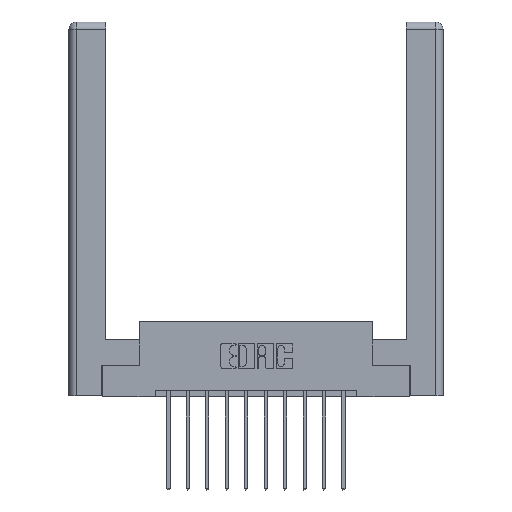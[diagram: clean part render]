
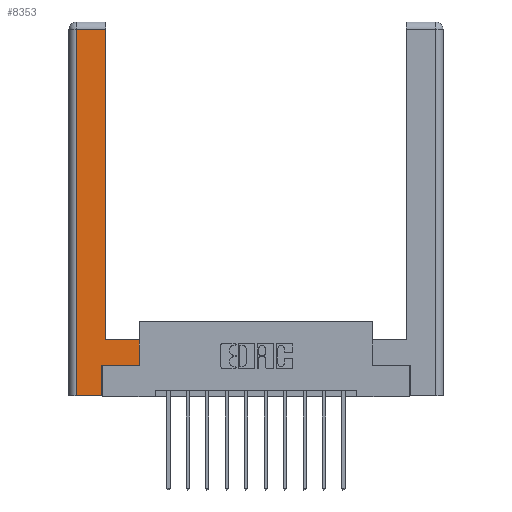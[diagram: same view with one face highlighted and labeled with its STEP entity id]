
A CAD part, top view. The second image highlights one B-rep face of the part: STEP entity #8353.
In plain terms, the highlighted planar face has unit normal (0, 0, 1).
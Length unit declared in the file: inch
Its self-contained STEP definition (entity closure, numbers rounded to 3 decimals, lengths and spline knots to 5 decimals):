
#63 = EDGE_LOOP ( 'NONE', ( #5025, #578, #2762, #4601, #14393, #1613, #6290, #5236 ) ) ;
#109 = DIRECTION ( 'NONE',  ( 0., 1., 0. ) ) ;
#138 = DIRECTION ( 'NONE',  ( 0., 1., 0. ) ) ;
#261 = DIRECTION ( 'NONE',  ( 1., 0., 0. ) ) ;
#522 = LINE ( 'NONE', #3432, #3669 ) ;
#578 = ORIENTED_EDGE ( 'NONE', *, *, #1402, .T. ) ;
#630 = VECTOR ( 'NONE', #9460, 39.37008 ) ;
#1001 = VECTOR ( 'NONE', #12050, 39.37008 ) ;
#1402 = EDGE_CURVE ( 'NONE', #11550, #8214, #7752, .T. ) ;
#1460 = CARTESIAN_POINT ( 'NONE',  ( 0.295, 0.45, 0. ) ) ;
#1613 = ORIENTED_EDGE ( 'NONE', *, *, #5504, .T. ) ;
#1838 = VECTOR ( 'NONE', #261, 39.37008 ) ;
#2034 = EDGE_CURVE ( 'NONE', #13854, #13527, #8766, .T. ) ;
#2553 = DIRECTION ( 'NONE',  ( -1., 0., 0. ) ) ;
#2762 = ORIENTED_EDGE ( 'NONE', *, *, #7700, .T. ) ;
#3165 = CARTESIAN_POINT ( 'NONE',  ( 0.265, 0., 0. ) ) ;
#3342 = CARTESIAN_POINT ( 'NONE',  ( 0.295, 3., 0. ) ) ;
#3417 = LINE ( 'NONE', #1460, #630 ) ;
#3432 = CARTESIAN_POINT ( 'NONE',  ( 0.565, 0.45, 0. ) ) ;
#3496 = CARTESIAN_POINT ( 'NONE',  ( 0.565, 0.245, 0. ) ) ;
#3533 = CARTESIAN_POINT ( 'NONE',  ( 0.0615, 2.94, 0. ) ) ;
#3669 = VECTOR ( 'NONE', #9099, 39.37008 ) ;
#3971 = CARTESIAN_POINT ( 'NONE',  ( 0.265, 0., 0. ) ) ;
#4296 = EDGE_CURVE ( 'NONE', #12742, #10742, #3417, .T. ) ;
#4601 = ORIENTED_EDGE ( 'NONE', *, *, #2034, .T. ) ;
#4670 = LINE ( 'NONE', #13049, #1001 ) ;
#4838 = CARTESIAN_POINT ( 'NONE',  ( 0.0615, 2.94, 0. ) ) ;
#5025 = ORIENTED_EDGE ( 'NONE', *, *, #7947, .T. ) ;
#5092 = VECTOR ( 'NONE', #138, 39.37008 ) ;
#5236 = ORIENTED_EDGE ( 'NONE', *, *, #4296, .T. ) ;
#5504 = EDGE_CURVE ( 'NONE', #6971, #14296, #6433, .T. ) ;
#5988 = PLANE ( 'NONE',  #8717 ) ;
#6191 = CARTESIAN_POINT ( 'NONE',  ( 0.295, 0.45, 0. ) ) ;
#6290 = ORIENTED_EDGE ( 'NONE', *, *, #12501, .T. ) ;
#6350 = CARTESIAN_POINT ( 'NONE',  ( 0.0615, 0., 0. ) ) ;
#6433 = LINE ( 'NONE', #13715, #1838 ) ;
#6971 = VERTEX_POINT ( 'NONE', #14559 ) ;
#6976 = FACE_OUTER_BOUND ( 'NONE', #63, .T. ) ;
#7532 = LINE ( 'NONE', #3342, #7866 ) ;
#7700 = EDGE_CURVE ( 'NONE', #8214, #13854, #4670, .T. ) ;
#7752 = LINE ( 'NONE', #4838, #8796 ) ;
#7866 = VECTOR ( 'NONE', #109, 39.37008 ) ;
#7947 = EDGE_CURVE ( 'NONE', #10742, #11550, #7532, .T. ) ;
#8214 = VERTEX_POINT ( 'NONE', #3533 ) ;
#8335 = CARTESIAN_POINT ( 'NONE',  ( 0.295, 2.94, 0. ) ) ;
#8353 = ADVANCED_FACE ( 'NONE', ( #6976 ), #5988, .F. ) ;
#8717 = AXIS2_PLACEMENT_3D ( 'NONE', #10618, #11653, #2553 ) ;
#8766 = LINE ( 'NONE', #3971, #13172 ) ;
#8796 = VECTOR ( 'NONE', #14194, 39.37008 ) ;
#9099 = DIRECTION ( 'NONE',  ( 0., 1., 0. ) ) ;
#9460 = DIRECTION ( 'NONE',  ( -1., 0., 0. ) ) ;
#10618 = CARTESIAN_POINT ( 'NONE',  ( 0., 0., 0. ) ) ;
#10742 = VERTEX_POINT ( 'NONE', #6191 ) ;
#11064 = LINE ( 'NONE', #12473, #5092 ) ;
#11550 = VERTEX_POINT ( 'NONE', #8335 ) ;
#11653 = DIRECTION ( 'NONE',  ( 0., 0., -1. ) ) ;
#12050 = DIRECTION ( 'NONE',  ( 0., -1., 0. ) ) ;
#12283 = EDGE_CURVE ( 'NONE', #13527, #6971, #11064, .T. ) ;
#12473 = CARTESIAN_POINT ( 'NONE',  ( 0.265, 0.245, 0. ) ) ;
#12501 = EDGE_CURVE ( 'NONE', #14296, #12742, #522, .T. ) ;
#12742 = VERTEX_POINT ( 'NONE', #14515 ) ;
#13049 = CARTESIAN_POINT ( 'NONE',  ( 0.0615, 0., 0. ) ) ;
#13172 = VECTOR ( 'NONE', #13177, 39.37008 ) ;
#13177 = DIRECTION ( 'NONE',  ( 1., 0., 0. ) ) ;
#13527 = VERTEX_POINT ( 'NONE', #3165 ) ;
#13715 = CARTESIAN_POINT ( 'NONE',  ( 0.565, 0.245, 0. ) ) ;
#13854 = VERTEX_POINT ( 'NONE', #6350 ) ;
#14194 = DIRECTION ( 'NONE',  ( -1., 0., 0. ) ) ;
#14296 = VERTEX_POINT ( 'NONE', #3496 ) ;
#14393 = ORIENTED_EDGE ( 'NONE', *, *, #12283, .T. ) ;
#14515 = CARTESIAN_POINT ( 'NONE',  ( 0.565, 0.45, 0. ) ) ;
#14559 = CARTESIAN_POINT ( 'NONE',  ( 0.265, 0.245, 0. ) ) ;
